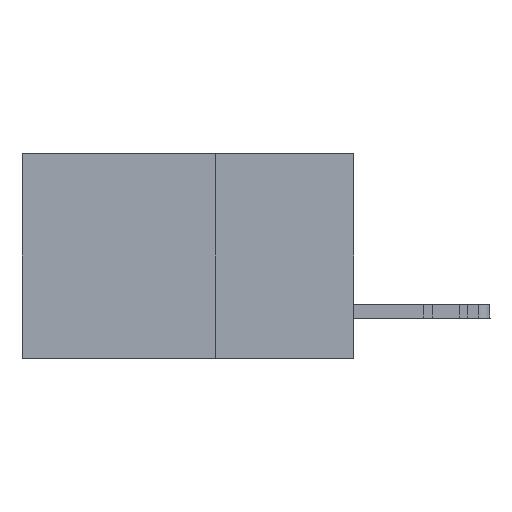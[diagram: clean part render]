
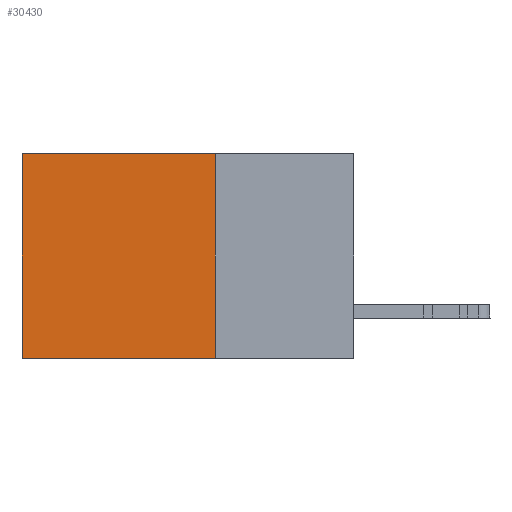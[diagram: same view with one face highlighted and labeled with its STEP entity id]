
A CAD part, left-side view. The second image highlights one B-rep face of the part: STEP entity #30430.
In plain terms, the highlighted planar face has unit normal (-1, 0, 0).
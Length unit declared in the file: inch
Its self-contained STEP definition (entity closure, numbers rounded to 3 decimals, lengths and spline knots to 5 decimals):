
#3021 = LINE ( 'NONE', #17363, #6307 ) ;
#4528 = LINE ( 'NONE', #35669, #35608 ) ;
#5110 = CARTESIAN_POINT ( 'NONE',  ( 0.2875, 0.25, -0.37 ) ) ;
#6162 = CARTESIAN_POINT ( 'NONE',  ( 0.2875, 0.25, 0. ) ) ;
#6307 = VECTOR ( 'NONE', #7560, 39.37008 ) ;
#7560 = DIRECTION ( 'NONE',  ( 0., 0., -1. ) ) ;
#9728 = DIRECTION ( 'NONE',  ( 0., 0., -1. ) ) ;
#11192 = DIRECTION ( 'NONE',  ( 0., 1., 0. ) ) ;
#11493 = VERTEX_POINT ( 'NONE', #5110 ) ;
#11644 = CARTESIAN_POINT ( 'NONE',  ( 0.2875, 0.25, -0.37 ) ) ;
#11750 = ORIENTED_EDGE ( 'NONE', *, *, #36806, .F. ) ;
#13317 = EDGE_CURVE ( 'NONE', #24592, #11493, #23345, .T. ) ;
#14031 = CARTESIAN_POINT ( 'NONE',  ( 0.2875, 0.25, 0. ) ) ;
#17363 = CARTESIAN_POINT ( 'NONE',  ( 0.2875, 0.6, 0. ) ) ;
#18670 = ORIENTED_EDGE ( 'NONE', *, *, #21415, .T. ) ;
#19394 = CARTESIAN_POINT ( 'NONE',  ( 0.2875, 0.6, -0.37 ) ) ;
#20092 = DIRECTION ( 'NONE',  ( 1., 0., 0. ) ) ;
#21145 = VECTOR ( 'NONE', #41861, 39.37008 ) ;
#21415 = EDGE_CURVE ( 'NONE', #33800, #40242, #3021, .T. ) ;
#23345 = LINE ( 'NONE', #14031, #21145 ) ;
#24592 = VERTEX_POINT ( 'NONE', #29866 ) ;
#26131 = DIRECTION ( 'NONE',  ( 0., 1., 0. ) ) ;
#27975 = FACE_OUTER_BOUND ( 'NONE', #36634, .T. ) ;
#29866 = CARTESIAN_POINT ( 'NONE',  ( 0.2875, 0.25, 0. ) ) ;
#30430 = ADVANCED_FACE ( 'NONE', ( #27975 ), #34787, .F. ) ;
#33800 = VERTEX_POINT ( 'NONE', #38526 ) ;
#34787 = PLANE ( 'NONE',  #38023 ) ;
#35062 = ORIENTED_EDGE ( 'NONE', *, *, #35109, .T. ) ;
#35109 = EDGE_CURVE ( 'NONE', #24592, #33800, #4528, .T. ) ;
#35608 = VECTOR ( 'NONE', #11192, 39.37008 ) ;
#35669 = CARTESIAN_POINT ( 'NONE',  ( 0.2875, 0.25, 0. ) ) ;
#36164 = LINE ( 'NONE', #11644, #37286 ) ;
#36634 = EDGE_LOOP ( 'NONE', ( #18670, #11750, #39040, #35062 ) ) ;
#36806 = EDGE_CURVE ( 'NONE', #11493, #40242, #36164, .T. ) ;
#37286 = VECTOR ( 'NONE', #26131, 39.37008 ) ;
#38023 = AXIS2_PLACEMENT_3D ( 'NONE', #6162, #20092, #9728 ) ;
#38526 = CARTESIAN_POINT ( 'NONE',  ( 0.2875, 0.6, 0. ) ) ;
#39040 = ORIENTED_EDGE ( 'NONE', *, *, #13317, .F. ) ;
#40242 = VERTEX_POINT ( 'NONE', #19394 ) ;
#41861 = DIRECTION ( 'NONE',  ( 0., 0., -1. ) ) ;
